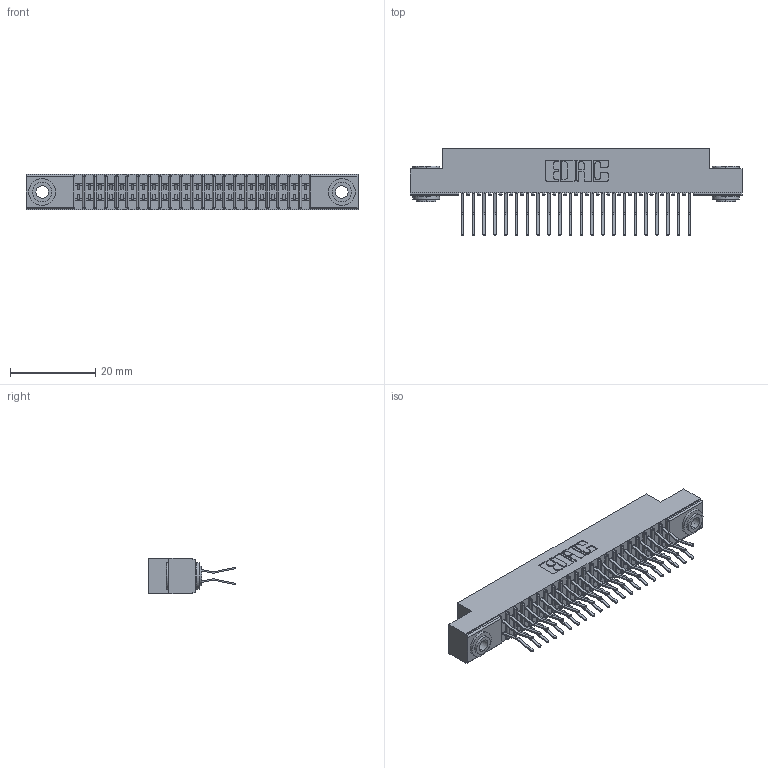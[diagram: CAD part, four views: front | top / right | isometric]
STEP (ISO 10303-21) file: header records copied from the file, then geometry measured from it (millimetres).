
FILE_DESCRIPTION (( 'STEP AP203' ), '1' );
FILE_NAME ('391-044-560-203.STEP', '2018-08-09T02:46:28', ( '' ), ( '' ), 'SwSTEP 2.0', 'SolidWorks 2016', '' );
FILE_SCHEMA (( 'CONFIG_CONTROL_DESIGN' ));
Length unit declared in the file: inch
Products named in the file (4): 341 Part_.156 (3.96) Dia Mounting Holes; 341-292-001_341-292-160; 345-250-002_345-250-002-102; 391-044-560-203
Assembly tree (47 placements, depth 2):
  391-044-560-203
    341 Part_.156 (3.96) Dia Mounting Holes
    341-292-001_341-292-160  x44
    345-250-002_345-250-002-102  x2
Bounding box: 78.11 x 20.37 x 8.38 mm (x, y, z)
Volume: 4491.6 mm3; surface area: 9911 mm2
Topology: 47 solids, 47 shells, 3248 faces, 9382 edges, 6086 vertices
Faces by surface type: plane 1852, cylinder 1300, sphere 46, torus 42, cone 8
Entity records: 30494 total; most frequent: CARTESIAN_POINT 5051, ORIENTED_EDGE 5008, DIRECTION 4936, EDGE_CURVE 2504, VECTOR 1986, LINE 1986, VERTEX_POINT 1590, AXIS2_PLACEMENT_3D 1475
